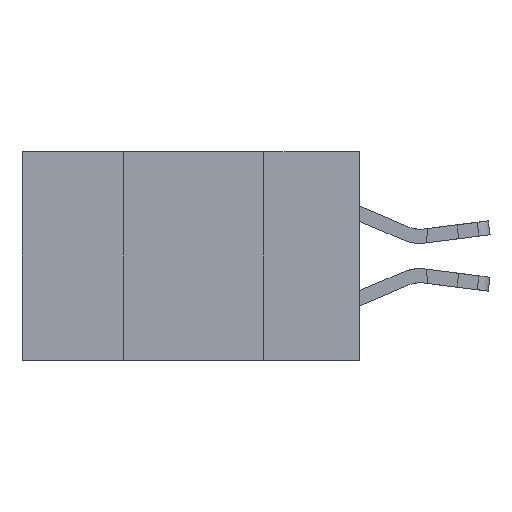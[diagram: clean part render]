
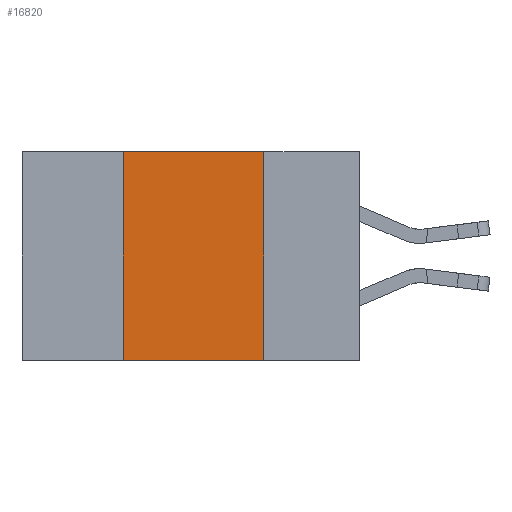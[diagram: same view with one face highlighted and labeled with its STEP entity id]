
A CAD part, left-side view. The second image highlights one B-rep face of the part: STEP entity #16820.
In plain terms, the highlighted planar face has unit normal (-1, 0, 0).
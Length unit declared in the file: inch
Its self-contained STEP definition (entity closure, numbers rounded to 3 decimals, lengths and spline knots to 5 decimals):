
#703 = ORIENTED_EDGE ( 'NONE', *, *, #23891, .F. ) ;
#977 = CARTESIAN_POINT ( 'NONE',  ( 0., 0.42, 0. ) ) ;
#1415 = CARTESIAN_POINT ( 'NONE',  ( 0., 0.6, 0. ) ) ;
#1709 = CARTESIAN_POINT ( 'NONE',  ( 0., 0.17, 0. ) ) ;
#5991 = DIRECTION ( 'NONE',  ( 0., -1., 0. ) ) ;
#6351 = CARTESIAN_POINT ( 'NONE',  ( 0., 0.17, 0. ) ) ;
#6472 = PLANE ( 'NONE',  #16296 ) ;
#7233 = LINE ( 'NONE', #18569, #12277 ) ;
#7811 = CARTESIAN_POINT ( 'NONE',  ( 0., 0.6, 0. ) ) ;
#8687 = VECTOR ( 'NONE', #5991, 39.37008 ) ;
#8699 = DIRECTION ( 'NONE',  ( 0., -1., 0. ) ) ;
#8806 = FACE_OUTER_BOUND ( 'NONE', #21794, .T. ) ;
#8996 = LINE ( 'NONE', #6351, #9615 ) ;
#9408 = ORIENTED_EDGE ( 'NONE', *, *, #12505, .F. ) ;
#9615 = VECTOR ( 'NONE', #14075, 39.37008 ) ;
#9969 = EDGE_CURVE ( 'NONE', #15267, #27659, #7233, .T. ) ;
#11428 = DIRECTION ( 'NONE',  ( 0., 0., 1. ) ) ;
#12277 = VECTOR ( 'NONE', #11428, 39.37008 ) ;
#12505 = EDGE_CURVE ( 'NONE', #27659, #17662, #22657, .T. ) ;
#13118 = CARTESIAN_POINT ( 'NONE',  ( 0., 0.17, -0.37 ) ) ;
#14075 = DIRECTION ( 'NONE',  ( 0., 0., -1. ) ) ;
#15267 = VERTEX_POINT ( 'NONE', #19772 ) ;
#15748 = ORIENTED_EDGE ( 'NONE', *, *, #29944, .T. ) ;
#16296 = AXIS2_PLACEMENT_3D ( 'NONE', #7811, #17254, #19585 ) ;
#16820 = ADVANCED_FACE ( 'NONE', ( #8806 ), #6472, .F. ) ;
#17254 = DIRECTION ( 'NONE',  ( 1., 0., 0. ) ) ;
#17662 = VERTEX_POINT ( 'NONE', #1709 ) ;
#18569 = CARTESIAN_POINT ( 'NONE',  ( 0., 0.42, 0. ) ) ;
#19585 = DIRECTION ( 'NONE',  ( 0., 0., -1. ) ) ;
#19772 = CARTESIAN_POINT ( 'NONE',  ( 0., 0.42, -0.37 ) ) ;
#21180 = VECTOR ( 'NONE', #8699, 39.37008 ) ;
#21494 = ORIENTED_EDGE ( 'NONE', *, *, #9969, .F. ) ;
#21794 = EDGE_LOOP ( 'NONE', ( #703, #9408, #21494, #15748 ) ) ;
#22435 = VERTEX_POINT ( 'NONE', #13118 ) ;
#22657 = LINE ( 'NONE', #1415, #21180 ) ;
#23891 = EDGE_CURVE ( 'NONE', #17662, #22435, #8996, .T. ) ;
#27232 = CARTESIAN_POINT ( 'NONE',  ( 0., 0.6, -0.37 ) ) ;
#27659 = VERTEX_POINT ( 'NONE', #977 ) ;
#29553 = LINE ( 'NONE', #27232, #8687 ) ;
#29944 = EDGE_CURVE ( 'NONE', #15267, #22435, #29553, .T. ) ;
